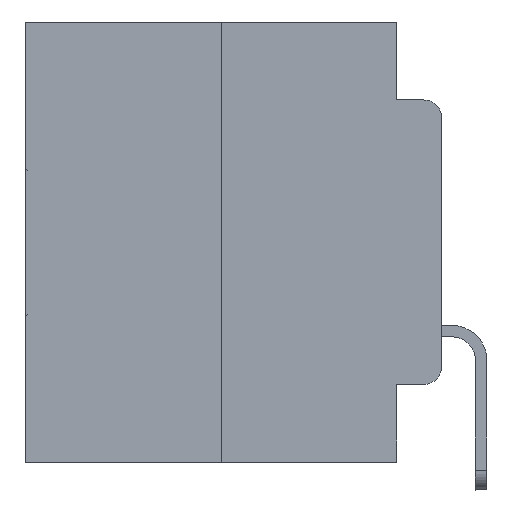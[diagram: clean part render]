
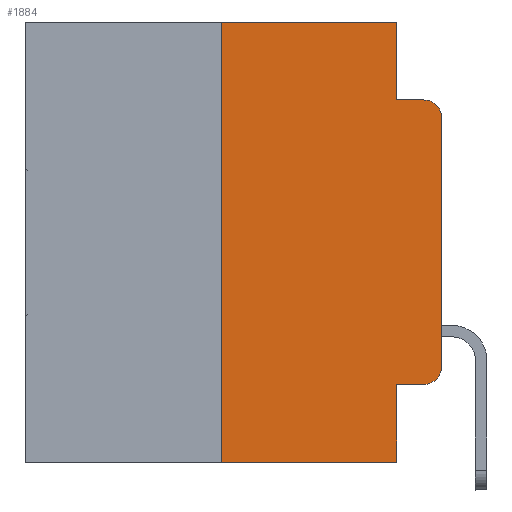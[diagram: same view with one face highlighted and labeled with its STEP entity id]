
A CAD part, left-side view. The second image highlights one B-rep face of the part: STEP entity #1884.
In plain terms, the highlighted planar face has unit normal (-1, 0, 0).
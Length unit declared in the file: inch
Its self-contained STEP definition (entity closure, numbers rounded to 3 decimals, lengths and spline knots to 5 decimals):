
#379 = ORIENTED_EDGE ( 'NONE', *, *, #23199, .T. ) ;
#449 = CARTESIAN_POINT ( 'NONE',  ( 0., 0.051, -0.4115 ) ) ;
#508 = EDGE_CURVE ( 'NONE', #20702, #7789, #8115, .T. ) ;
#634 = VERTEX_POINT ( 'NONE', #26168 ) ;
#653 = DIRECTION ( 'NONE',  ( 1., 0., 0. ) ) ;
#864 = CARTESIAN_POINT ( 'NONE',  ( 0., 0., -0.1085 ) ) ;
#1407 = VERTEX_POINT ( 'NONE', #864 ) ;
#1808 = CARTESIAN_POINT ( 'NONE',  ( 0., 0., -0.3915 ) ) ;
#1884 = ADVANCED_FACE ( 'NONE', ( #5310 ), #27443, .F. ) ;
#2613 = VECTOR ( 'NONE', #23044, 39.37008 ) ;
#2632 = ORIENTED_EDGE ( 'NONE', *, *, #13722, .F. ) ;
#3384 = VERTEX_POINT ( 'NONE', #23424 ) ;
#3440 = ORIENTED_EDGE ( 'NONE', *, *, #23935, .T. ) ;
#3609 = VECTOR ( 'NONE', #28413, 39.37008 ) ;
#3719 = EDGE_CURVE ( 'NONE', #634, #7789, #23491, .T. ) ;
#4347 = EDGE_CURVE ( 'NONE', #11872, #21827, #19811, .T. ) ;
#4474 = CARTESIAN_POINT ( 'NONE',  ( 0., 0.25, 0. ) ) ;
#5058 = DIRECTION ( 'NONE',  ( 0., -1., 0. ) ) ;
#5310 = FACE_OUTER_BOUND ( 'NONE', #27881, .T. ) ;
#5889 = EDGE_CURVE ( 'NONE', #21827, #3384, #20906, .T. ) ;
#6053 = DIRECTION ( 'NONE',  ( 0., 0., -1. ) ) ;
#6902 = CARTESIAN_POINT ( 'NONE',  ( 0., 0.02, -0.0885 ) ) ;
#7031 = VERTEX_POINT ( 'NONE', #6902 ) ;
#7210 = CARTESIAN_POINT ( 'NONE',  ( 0., 0.473, 0. ) ) ;
#7550 = LINE ( 'NONE', #16147, #17772 ) ;
#7618 = AXIS2_PLACEMENT_3D ( 'NONE', #7210, #653, #22661 ) ;
#7789 = VERTEX_POINT ( 'NONE', #21730 ) ;
#8115 = LINE ( 'NONE', #18820, #2613 ) ;
#8313 = ORIENTED_EDGE ( 'NONE', *, *, #4347, .F. ) ;
#8376 = ORIENTED_EDGE ( 'NONE', *, *, #3719, .T. ) ;
#8704 = AXIS2_PLACEMENT_3D ( 'NONE', #17794, #22309, #11217 ) ;
#8945 = ORIENTED_EDGE ( 'NONE', *, *, #10773, .F. ) ;
#10773 = EDGE_CURVE ( 'NONE', #634, #11872, #24441, .T. ) ;
#11217 = DIRECTION ( 'NONE',  ( 0., 0., -1. ) ) ;
#11697 = DIRECTION ( 'NONE',  ( 0., 0., -1. ) ) ;
#11872 = VERTEX_POINT ( 'NONE', #17462 ) ;
#11985 = CARTESIAN_POINT ( 'NONE',  ( 0., 0.051, 0. ) ) ;
#12094 = AXIS2_PLACEMENT_3D ( 'NONE', #25735, #19047, #6053 ) ;
#12180 = EDGE_CURVE ( 'NONE', #24154, #20328, #24652, .T. ) ;
#12320 = VECTOR ( 'NONE', #21375, 39.37008 ) ;
#12869 = CIRCLE ( 'NONE', #8704, 0.02 ) ;
#13363 = DIRECTION ( 'NONE',  ( 0., 0., 1. ) ) ;
#13722 = EDGE_CURVE ( 'NONE', #3384, #7031, #7550, .T. ) ;
#13870 = VECTOR ( 'NONE', #11697, 39.37008 ) ;
#14155 = DIRECTION ( 'NONE',  ( 0., -1., 0. ) ) ;
#16147 = CARTESIAN_POINT ( 'NONE',  ( 0., 0.051, -0.0885 ) ) ;
#16700 = ORIENTED_EDGE ( 'NONE', *, *, #12180, .T. ) ;
#17462 = CARTESIAN_POINT ( 'NONE',  ( 0., 0.25, 0. ) ) ;
#17772 = VECTOR ( 'NONE', #5058, 39.37008 ) ;
#17794 = CARTESIAN_POINT ( 'NONE',  ( 0., 0.02, -0.1085 ) ) ;
#17841 = ORIENTED_EDGE ( 'NONE', *, *, #508, .F. ) ;
#18634 = VECTOR ( 'NONE', #13363, 39.37008 ) ;
#18820 = CARTESIAN_POINT ( 'NONE',  ( 0., 0.051, 0. ) ) ;
#18835 = LINE ( 'NONE', #449, #27702 ) ;
#19047 = DIRECTION ( 'NONE',  ( -1., 0., 0. ) ) ;
#19276 = ORIENTED_EDGE ( 'NONE', *, *, #5889, .F. ) ;
#19811 = LINE ( 'NONE', #28662, #27349 ) ;
#20328 = VERTEX_POINT ( 'NONE', #1808 ) ;
#20545 = CARTESIAN_POINT ( 'NONE',  ( 0., 0.051, -0.4115 ) ) ;
#20702 = VERTEX_POINT ( 'NONE', #20545 ) ;
#20906 = LINE ( 'NONE', #11985, #13870 ) ;
#21219 = ORIENTED_EDGE ( 'NONE', *, *, #25604, .T. ) ;
#21375 = DIRECTION ( 'NONE',  ( 0., 0., 1. ) ) ;
#21467 = CARTESIAN_POINT ( 'NONE',  ( 0., 0.473, -0.5 ) ) ;
#21730 = CARTESIAN_POINT ( 'NONE',  ( 0., 0.051, -0.5 ) ) ;
#21827 = VERTEX_POINT ( 'NONE', #22831 ) ;
#22309 = DIRECTION ( 'NONE',  ( -1., 0., 0. ) ) ;
#22661 = DIRECTION ( 'NONE',  ( 0., 0., -1. ) ) ;
#22831 = CARTESIAN_POINT ( 'NONE',  ( 0., 0.051, 0. ) ) ;
#23044 = DIRECTION ( 'NONE',  ( 0., 0., -1. ) ) ;
#23199 = EDGE_CURVE ( 'NONE', #20328, #1407, #28054, .T. ) ;
#23424 = CARTESIAN_POINT ( 'NONE',  ( 0., 0.051, -0.0885 ) ) ;
#23491 = LINE ( 'NONE', #21467, #3609 ) ;
#23910 = CARTESIAN_POINT ( 'NONE',  ( 0., 0.02, -0.4115 ) ) ;
#23935 = EDGE_CURVE ( 'NONE', #20702, #24154, #18835, .T. ) ;
#24025 = DIRECTION ( 'NONE',  ( 0., -1., 0. ) ) ;
#24154 = VERTEX_POINT ( 'NONE', #23910 ) ;
#24441 = LINE ( 'NONE', #4474, #18634 ) ;
#24652 = CIRCLE ( 'NONE', #12094, 0.02 ) ;
#25604 = EDGE_CURVE ( 'NONE', #1407, #7031, #12869, .T. ) ;
#25735 = CARTESIAN_POINT ( 'NONE',  ( 0., 0.02, -0.3915 ) ) ;
#26147 = CARTESIAN_POINT ( 'NONE',  ( 0., 0., 0. ) ) ;
#26168 = CARTESIAN_POINT ( 'NONE',  ( 0., 0.25, -0.5 ) ) ;
#27349 = VECTOR ( 'NONE', #24025, 39.37008 ) ;
#27443 = PLANE ( 'NONE',  #7618 ) ;
#27702 = VECTOR ( 'NONE', #14155, 39.37008 ) ;
#27881 = EDGE_LOOP ( 'NONE', ( #379, #21219, #2632, #19276, #8313, #8945, #8376, #17841, #3440, #16700 ) ) ;
#28054 = LINE ( 'NONE', #26147, #12320 ) ;
#28413 = DIRECTION ( 'NONE',  ( 0., -1., 0. ) ) ;
#28662 = CARTESIAN_POINT ( 'NONE',  ( 0., 0.473, 0. ) ) ;
